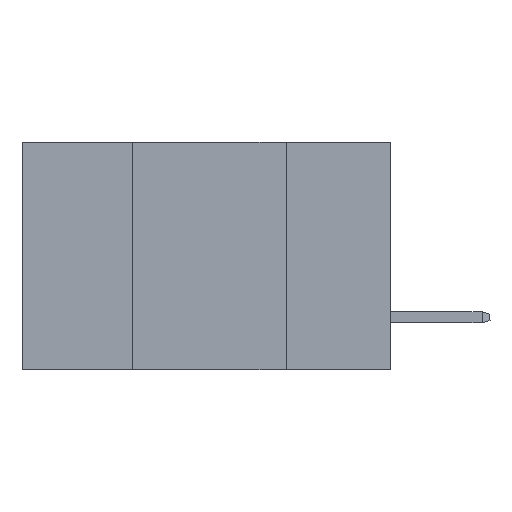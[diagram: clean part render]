
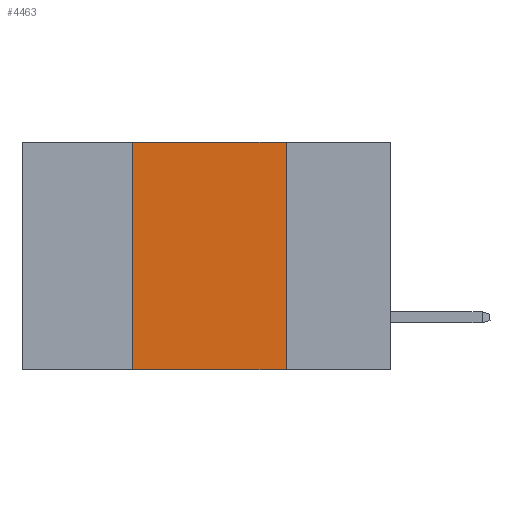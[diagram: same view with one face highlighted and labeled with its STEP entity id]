
A CAD part, left-side view. The second image highlights one B-rep face of the part: STEP entity #4463.
In plain terms, the highlighted planar face has unit normal (-1, 0, 0).
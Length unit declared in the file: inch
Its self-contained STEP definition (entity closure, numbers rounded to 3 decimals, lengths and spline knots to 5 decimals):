
#1119 = DIRECTION ( 'NONE',  ( 0., -1., 0. ) ) ;
#3101 = FACE_OUTER_BOUND ( 'NONE', #6043, .T. ) ;
#4246 = ORIENTED_EDGE ( 'NONE', *, *, #7785, .F. ) ;
#4431 = VERTEX_POINT ( 'NONE', #12742 ) ;
#4463 = ADVANCED_FACE ( 'NONE', ( #3101 ), #10749, .F. ) ;
#5835 = EDGE_CURVE ( 'NONE', #7325, #18995, #16343, .T. ) ;
#6043 = EDGE_LOOP ( 'NONE', ( #15327, #10770, #4246, #17870 ) ) ;
#7325 = VERTEX_POINT ( 'NONE', #22452 ) ;
#7785 = EDGE_CURVE ( 'NONE', #12465, #7325, #21121, .T. ) ;
#8794 = CARTESIAN_POINT ( 'NONE',  ( 0., 0.6, -0.37 ) ) ;
#9614 = CARTESIAN_POINT ( 'NONE',  ( 0., 0.17, 0. ) ) ;
#10749 = PLANE ( 'NONE',  #18708 ) ;
#10770 = ORIENTED_EDGE ( 'NONE', *, *, #5835, .F. ) ;
#11331 = EDGE_CURVE ( 'NONE', #18995, #4431, #12988, .T. ) ;
#11495 = CARTESIAN_POINT ( 'NONE',  ( 0., 0.6, 0. ) ) ;
#11697 = DIRECTION ( 'NONE',  ( 0., 0., -1. ) ) ;
#11713 = DIRECTION ( 'NONE',  ( 0., 0., 1. ) ) ;
#12465 = VERTEX_POINT ( 'NONE', #17729 ) ;
#12742 = CARTESIAN_POINT ( 'NONE',  ( 0., 0.17, -0.37 ) ) ;
#12834 = DIRECTION ( 'NONE',  ( 0., 0., -1. ) ) ;
#12988 = LINE ( 'NONE', #9614, #23944 ) ;
#15327 = ORIENTED_EDGE ( 'NONE', *, *, #11331, .F. ) ;
#15672 = VECTOR ( 'NONE', #1119, 39.37008 ) ;
#15795 = LINE ( 'NONE', #8794, #20003 ) ;
#16343 = LINE ( 'NONE', #11495, #15672 ) ;
#17729 = CARTESIAN_POINT ( 'NONE',  ( 0., 0.42, -0.37 ) ) ;
#17870 = ORIENTED_EDGE ( 'NONE', *, *, #22553, .T. ) ;
#18708 = AXIS2_PLACEMENT_3D ( 'NONE', #23137, #25159, #12834 ) ;
#18995 = VERTEX_POINT ( 'NONE', #25157 ) ;
#19138 = DIRECTION ( 'NONE',  ( 0., -1., 0. ) ) ;
#20003 = VECTOR ( 'NONE', #19138, 39.37008 ) ;
#20490 = VECTOR ( 'NONE', #11713, 39.37008 ) ;
#21121 = LINE ( 'NONE', #26131, #20490 ) ;
#22452 = CARTESIAN_POINT ( 'NONE',  ( 0., 0.42, 0. ) ) ;
#22553 = EDGE_CURVE ( 'NONE', #12465, #4431, #15795, .T. ) ;
#23137 = CARTESIAN_POINT ( 'NONE',  ( 0., 0.6, 0. ) ) ;
#23944 = VECTOR ( 'NONE', #11697, 39.37008 ) ;
#25157 = CARTESIAN_POINT ( 'NONE',  ( 0., 0.17, 0. ) ) ;
#25159 = DIRECTION ( 'NONE',  ( 1., 0., 0. ) ) ;
#26131 = CARTESIAN_POINT ( 'NONE',  ( 0., 0.42, 0. ) ) ;
